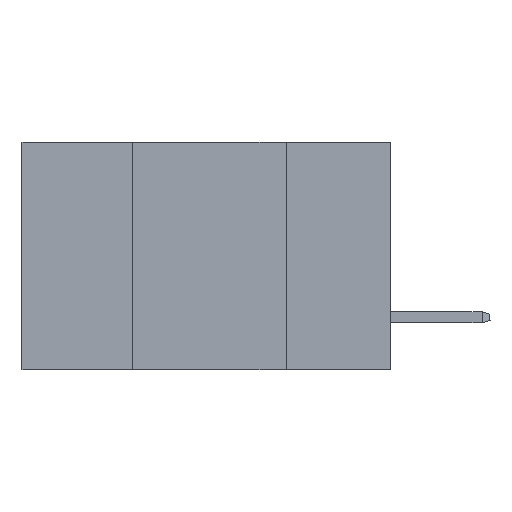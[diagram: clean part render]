
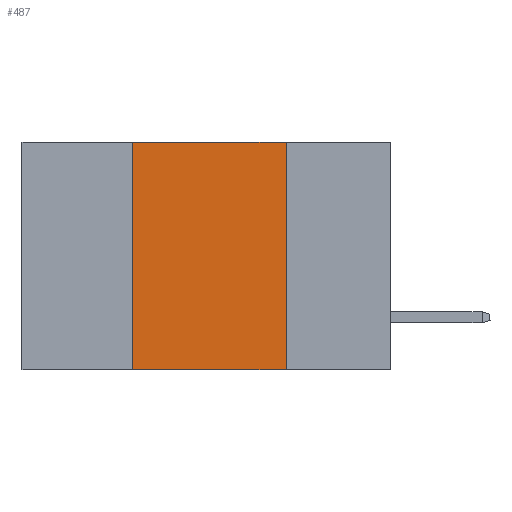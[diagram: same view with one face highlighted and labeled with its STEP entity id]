
A CAD part, left-side view. The second image highlights one B-rep face of the part: STEP entity #487.
In plain terms, the highlighted planar face has unit normal (-1, 0, 0).
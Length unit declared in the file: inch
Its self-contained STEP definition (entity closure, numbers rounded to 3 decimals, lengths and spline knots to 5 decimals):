
#95 = DIRECTION ( 'NONE',  ( 0., -1., 0. ) ) ;
#487 = ADVANCED_FACE ( 'NONE', ( #14858 ), #3693, .F. ) ;
#1216 = EDGE_LOOP ( 'NONE', ( #12736, #3440, #11097, #4773 ) ) ;
#1266 = DIRECTION ( 'NONE',  ( 0., 0., -1. ) ) ;
#1540 = DIRECTION ( 'NONE',  ( 0., 0., -1. ) ) ;
#1734 = CARTESIAN_POINT ( 'NONE',  ( 0., 0.17, -0.37 ) ) ;
#1858 = LINE ( 'NONE', #9375, #4751 ) ;
#2825 = DIRECTION ( 'NONE',  ( 0., 0., 1. ) ) ;
#2965 = CARTESIAN_POINT ( 'NONE',  ( 0., 0.42, 0. ) ) ;
#3134 = EDGE_CURVE ( 'NONE', #7703, #12288, #1858, .T. ) ;
#3306 = LINE ( 'NONE', #12299, #3484 ) ;
#3440 = ORIENTED_EDGE ( 'NONE', *, *, #9499, .F. ) ;
#3484 = VECTOR ( 'NONE', #95, 39.37008 ) ;
#3693 = PLANE ( 'NONE',  #7305 ) ;
#3862 = VECTOR ( 'NONE', #2825, 39.37008 ) ;
#3995 = VECTOR ( 'NONE', #5094, 39.37008 ) ;
#4751 = VECTOR ( 'NONE', #1266, 39.37008 ) ;
#4773 = ORIENTED_EDGE ( 'NONE', *, *, #8983, .T. ) ;
#5094 = DIRECTION ( 'NONE',  ( 0., -1., 0. ) ) ;
#5379 = CARTESIAN_POINT ( 'NONE',  ( 0., 0.6, 0. ) ) ;
#6952 = EDGE_CURVE ( 'NONE', #12624, #9295, #13604, .T. ) ;
#7282 = LINE ( 'NONE', #10080, #3995 ) ;
#7305 = AXIS2_PLACEMENT_3D ( 'NONE', #5379, #10282, #1540 ) ;
#7703 = VERTEX_POINT ( 'NONE', #10172 ) ;
#8983 = EDGE_CURVE ( 'NONE', #12624, #12288, #7282, .T. ) ;
#9295 = VERTEX_POINT ( 'NONE', #15257 ) ;
#9375 = CARTESIAN_POINT ( 'NONE',  ( 0., 0.17, 0. ) ) ;
#9499 = EDGE_CURVE ( 'NONE', #9295, #7703, #3306, .T. ) ;
#10080 = CARTESIAN_POINT ( 'NONE',  ( 0., 0.6, -0.37 ) ) ;
#10172 = CARTESIAN_POINT ( 'NONE',  ( 0., 0.17, 0. ) ) ;
#10282 = DIRECTION ( 'NONE',  ( 1., 0., 0. ) ) ;
#11097 = ORIENTED_EDGE ( 'NONE', *, *, #6952, .F. ) ;
#12288 = VERTEX_POINT ( 'NONE', #1734 ) ;
#12299 = CARTESIAN_POINT ( 'NONE',  ( 0., 0.6, 0. ) ) ;
#12624 = VERTEX_POINT ( 'NONE', #15697 ) ;
#12736 = ORIENTED_EDGE ( 'NONE', *, *, #3134, .F. ) ;
#13604 = LINE ( 'NONE', #2965, #3862 ) ;
#14858 = FACE_OUTER_BOUND ( 'NONE', #1216, .T. ) ;
#15257 = CARTESIAN_POINT ( 'NONE',  ( 0., 0.42, 0. ) ) ;
#15697 = CARTESIAN_POINT ( 'NONE',  ( 0., 0.42, -0.37 ) ) ;
